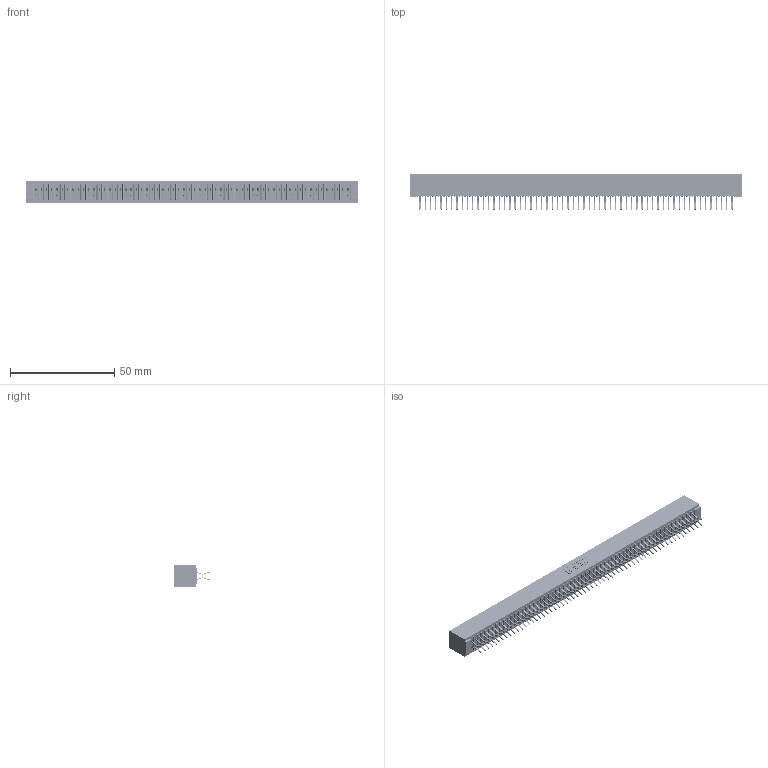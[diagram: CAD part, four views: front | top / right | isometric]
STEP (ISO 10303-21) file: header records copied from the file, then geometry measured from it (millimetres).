
FILE_DESCRIPTION (( 'STEP AP203' ), '1' );
FILE_NAME ('341-120-556-201.STEP', '2018-08-08T15:01:23', ( '' ), ( '' ), 'SwSTEP 2.0', 'SolidWorks 2016', '' );
FILE_SCHEMA (( 'CONFIG_CONTROL_DESIGN' ));
Length unit declared in the file: inch
Products named in the file (3): 341-292-001_341-292-156; 341-120-556-201; 341 Part_No Mounting Lugs
Assembly tree (121 placements, depth 2):
  341-120-556-201
    341 Part_No Mounting Lugs
    341-292-001_341-292-156  x120
Bounding box: 159.38 x 17.07 x 10.16 mm (x, y, z)
Volume: 12059.8 mm3; surface area: 22925 mm2
Topology: 121 solids, 121 shells, 8508 faces, 24712 edges, 16030 vertices
Faces by surface type: plane 4864, cylinder 3404, sphere 122, torus 118
Entity records: 70077 total; most frequent: CARTESIAN_POINT 11648, ORIENTED_EDGE 11576, DIRECTION 11294, EDGE_CURVE 5788, LINE 4694, VECTOR 4694, VERTEX_POINT 3654, AXIS2_PLACEMENT_3D 3300
